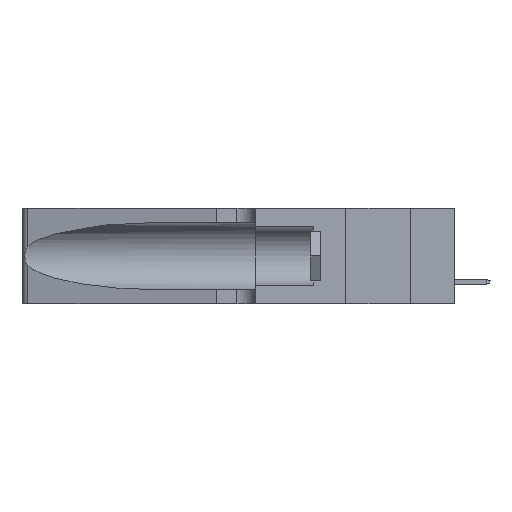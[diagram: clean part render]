
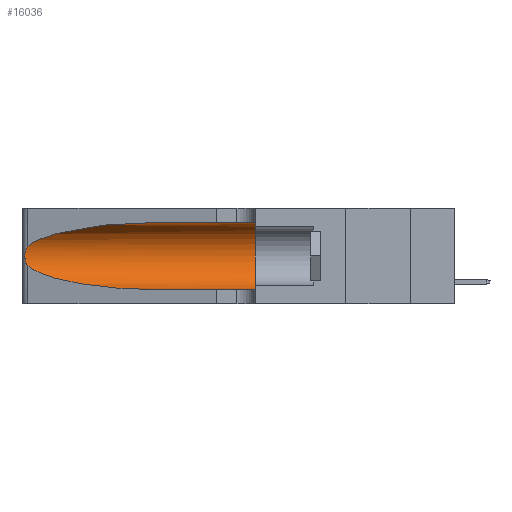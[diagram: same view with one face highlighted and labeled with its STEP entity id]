
A CAD part, left-side view. The second image highlights one B-rep face of the part: STEP entity #16036.
In plain terms, the highlighted cylindrical face has radius 3.308 mm (diameter 6.617 mm), a partial arc.
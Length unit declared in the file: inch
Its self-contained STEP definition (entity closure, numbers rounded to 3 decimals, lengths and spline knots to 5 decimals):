
#1526 = CARTESIAN_POINT ( 'NONE',  ( 0.26017, 1.23833, 0.17102 ) ) ;
#1748 = DIRECTION ( 'NONE',  ( 0., -1., 0. ) ) ;
#3025 = CARTESIAN_POINT ( 'NONE',  ( 0.2373, 1.15595, 0.28018 ) ) ;
#3431 = CARTESIAN_POINT ( 'NONE',  ( 0.1305, 1.61858, 0.05475 ) ) ;
#3556 = CARTESIAN_POINT ( 'NONE',  ( 0.1305, 0.35, 0.05475 ) ) ;
#5234 = CARTESIAN_POINT ( 'NONE',  ( 0.25789, 1.23486, 0.15765 ) ) ;
#5501 = CARTESIAN_POINT ( 'NONE',  ( 0.25555, 1.22993, 0.14849 ) ) ;
#6033 = CARTESIAN_POINT ( 'NONE',  ( 0.26075, 1.23896, 0.19203 ) ) ;
#7141 = DIRECTION ( 'NONE',  ( 0., -1., 0. ) ) ;
#9501 = CARTESIAN_POINT ( 'NONE',  ( 0.26018, 1.23835, 0.19895 ) ) ;
#10520 = ORIENTED_EDGE ( 'NONE', *, *, #43356, .F. ) ;
#10606 = LINE ( 'NONE', #3431, #20422 ) ;
#10665 = CYLINDRICAL_SURFACE ( 'NONE', #35094, 0.13025 ) ;
#11019 = CARTESIAN_POINT ( 'NONE',  ( 0.25487, 1.22718, 0.14631 ) ) ;
#11185 = DIRECTION ( 'NONE',  ( 0., 0., -1. ) ) ;
#11976 = ORIENTED_EDGE ( 'NONE', *, *, #45694, .F. ) ;
#12196 = VERTEX_POINT ( 'NONE', #52202 ) ;
#14117 = CARTESIAN_POINT ( 'NONE',  ( 0.1305, 0.35, 0.185 ) ) ;
#14175 = EDGE_LOOP ( 'NONE', ( #41397, #43578, #51039, #25925, #10520, #11976 ) ) ;
#14367 = FACE_OUTER_BOUND ( 'NONE', #14175, .T. ) ;
#14882 = DIRECTION ( 'NONE',  ( 0., -1., 0. ) ) ;
#16036 = ADVANCED_FACE ( 'NONE', ( #14367 ), #10665, .F. ) ;
#17230 = VECTOR ( 'NONE', #1748, 39.37008 ) ;
#17675 = CARTESIAN_POINT ( 'NONE',  ( 0.1305, 1.61858, 0.31525 ) ) ;
#17708 = CARTESIAN_POINT ( 'NONE',  ( 0.25639, 1.23186, 0.15144 ) ) ;
#19222 = CARTESIAN_POINT ( 'NONE',  ( 0.25487, 1.22718, 0.22369 ) ) ;
#20196 = EDGE_CURVE ( 'NONE', #31728, #29500, #39075, .T. ) ;
#20422 = VECTOR ( 'NONE', #7141, 39.37008 ) ;
#21421 = CARTESIAN_POINT ( 'NONE',  ( 0.25487, 1.22718, 0.14631 ) ) ;
#22059 = VERTEX_POINT ( 'NONE', #3556 ) ;
#22229 = CARTESIAN_POINT ( 'NONE',  ( 0.25856, 1.23593, 0.16098 ) ) ;
#23884 = CARTESIAN_POINT ( 'NONE',  ( 0.25487, 1.22718, 0.14631 ) ) ;
#25925 = ORIENTED_EDGE ( 'NONE', *, *, #42479, .T. ) ;
#26782 = CARTESIAN_POINT ( 'NONE',  ( 0.1305, 0.72297, 0.05475 ) ) ;
#29500 = VERTEX_POINT ( 'NONE', #11019 ) ;
#30337 = DIRECTION ( 'NONE',  ( 0., 1., 0. ) ) ;
#30586 = CARTESIAN_POINT ( 'NONE',  ( 0.1305, 1.61858, 0.185 ) ) ;
#30635 = AXIS2_PLACEMENT_3D ( 'NONE', #14117, #30337, #46020 ) ;
#31728 = VERTEX_POINT ( 'NONE', #33934 ) ;
#31838 = CARTESIAN_POINT ( 'NONE',  ( 0.18966, 0.96281, 0.05475 ) ) ;
#33878 = LINE ( 'NONE', #17675, #17230 ) ;
#33934 = CARTESIAN_POINT ( 'NONE',  ( 0.25487, 1.22718, 0.22369 ) ) ;
#34432 = CARTESIAN_POINT ( 'NONE',  ( 0.25555, 1.22994, 0.2215 ) ) ;
#35094 = AXIS2_PLACEMENT_3D ( 'NONE', #30586, #14882, #11185 ) ;
#37906 = CARTESIAN_POINT ( 'NONE',  ( 0.25639, 1.23184, 0.21858 ) ) ;
#39075 = B_SPLINE_CURVE_WITH_KNOTS ( 'NONE', 3,
 ( #41628, #34432, #37906, #42429, #50647, #9501, #6033, #46397, #1526, #22229, #5234, #17708, #5501, #21421 ),
 .UNSPECIFIED., .F., .F.,
 ( 4, 2, 2, 2, 2, 2, 4 ),
 ( 0., 0.00027, 0.00053, 0.00107, 0.0016, 0.00187, 0.00214 ),
 .UNSPECIFIED. ) ;
#39145 = CIRCLE ( 'NONE', #30635, 0.13025 ) ;
#39435 = CARTESIAN_POINT ( 'NONE',  ( 0.18966, 0.96281, 0.31525 ) ) ;
#39580 = CARTESIAN_POINT ( 'NONE',  ( 0.2373, 1.15595, 0.08982 ) ) ;
#41063 =( BOUNDED_CURVE ( )  B_SPLINE_CURVE ( 3, ( #23884, #39580, #31838, #48064 ),
 .UNSPECIFIED., .F., .F. ) 
 B_SPLINE_CURVE_WITH_KNOTS ( ( 4, 4 ),
 ( 3.44316, 4.71239 ),
 .UNSPECIFIED. ) 
 CURVE ( )  GEOMETRIC_REPRESENTATION_ITEM ( )  RATIONAL_B_SPLINE_CURVE ( ( 1., 0.87, 0.87, 1. ) ) 
 REPRESENTATION_ITEM ( '' )  );
#41204 = VERTEX_POINT ( 'NONE', #26782 ) ;
#41397 = ORIENTED_EDGE ( 'NONE', *, *, #43058, .T. ) ;
#41628 = CARTESIAN_POINT ( 'NONE',  ( 0.25487, 1.22718, 0.22369 ) ) ;
#42429 = CARTESIAN_POINT ( 'NONE',  ( 0.25787, 1.23484, 0.2124 ) ) ;
#42479 = EDGE_CURVE ( 'NONE', #41204, #22059, #10606, .T. ) ;
#43058 = EDGE_CURVE ( 'NONE', #12196, #31728, #51917, .T. ) ;
#43356 = EDGE_CURVE ( 'NONE', #50390, #22059, #39145, .T. ) ;
#43578 = ORIENTED_EDGE ( 'NONE', *, *, #20196, .T. ) ;
#44172 = CARTESIAN_POINT ( 'NONE',  ( 0.1305, 0.72297, 0.31525 ) ) ;
#45694 = EDGE_CURVE ( 'NONE', #12196, #50390, #33878, .T. ) ;
#46020 = DIRECTION ( 'NONE',  ( 0., 0., 1. ) ) ;
#46365 = EDGE_CURVE ( 'NONE', #29500, #41204, #41063, .T. ) ;
#46397 = CARTESIAN_POINT ( 'NONE',  ( 0.26075, 1.23896, 0.178 ) ) ;
#46743 = CARTESIAN_POINT ( 'NONE',  ( 0.1305, 0.35, 0.31525 ) ) ;
#48064 = CARTESIAN_POINT ( 'NONE',  ( 0.1305, 0.72297, 0.05475 ) ) ;
#50390 = VERTEX_POINT ( 'NONE', #46743 ) ;
#50647 = CARTESIAN_POINT ( 'NONE',  ( 0.25854, 1.2359, 0.20912 ) ) ;
#51039 = ORIENTED_EDGE ( 'NONE', *, *, #46365, .T. ) ;
#51917 =( BOUNDED_CURVE ( )  B_SPLINE_CURVE ( 3, ( #44172, #39435, #3025, #19222 ),
 .UNSPECIFIED., .F., .T. ) 
 B_SPLINE_CURVE_WITH_KNOTS ( ( 4, 4 ),
 ( 1.5708, 2.84003 ),
 .UNSPECIFIED. ) 
 CURVE ( )  GEOMETRIC_REPRESENTATION_ITEM ( )  RATIONAL_B_SPLINE_CURVE ( ( 1., 0.87, 0.87, 1. ) ) 
 REPRESENTATION_ITEM ( '' )  );
#52202 = CARTESIAN_POINT ( 'NONE',  ( 0.1305, 0.72297, 0.31525 ) ) ;
